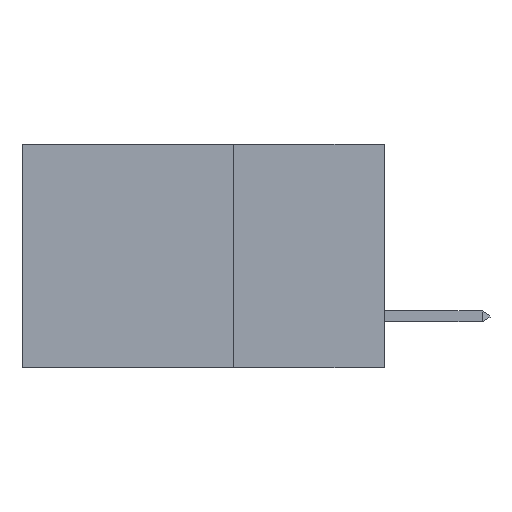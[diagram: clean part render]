
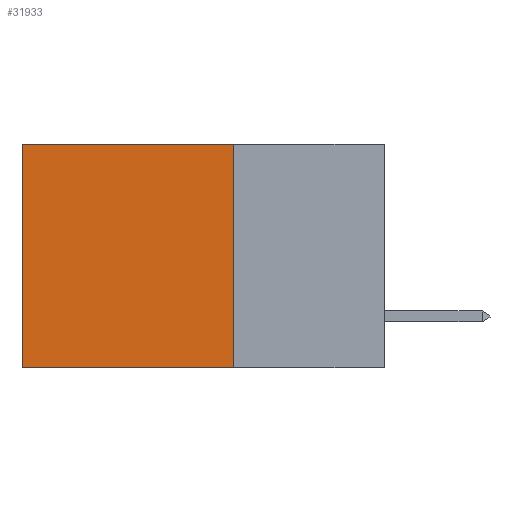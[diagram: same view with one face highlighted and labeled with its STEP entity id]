
A CAD part, left-side view. The second image highlights one B-rep face of the part: STEP entity #31933.
In plain terms, the highlighted planar face has unit normal (-1, 0, 0).
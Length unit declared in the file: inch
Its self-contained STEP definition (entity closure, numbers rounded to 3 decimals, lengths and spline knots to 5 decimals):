
#1397 = VERTEX_POINT ( 'NONE', #3713 ) ;
#1494 = DIRECTION ( 'NONE',  ( 0., 1., 0. ) ) ;
#3355 = DIRECTION ( 'NONE',  ( 0., 0., -1. ) ) ;
#3713 = CARTESIAN_POINT ( 'NONE',  ( 0.2875, 0.6, -0.37 ) ) ;
#4660 = VECTOR ( 'NONE', #1494, 39.37008 ) ;
#7984 = CARTESIAN_POINT ( 'NONE',  ( 0.2875, 0.6, 0. ) ) ;
#8040 = ORIENTED_EDGE ( 'NONE', *, *, #15448, .T. ) ;
#9040 = ORIENTED_EDGE ( 'NONE', *, *, #17969, .F. ) ;
#9834 = CARTESIAN_POINT ( 'NONE',  ( 0.2875, 0.25, -0.37 ) ) ;
#11094 = CARTESIAN_POINT ( 'NONE',  ( 0.2875, 0.6, 0. ) ) ;
#11198 = DIRECTION ( 'NONE',  ( 0., 0., -1. ) ) ;
#12249 = VERTEX_POINT ( 'NONE', #24648 ) ;
#13356 = VECTOR ( 'NONE', #24672, 39.37008 ) ;
#13552 = VECTOR ( 'NONE', #27266, 39.37008 ) ;
#14131 = CARTESIAN_POINT ( 'NONE',  ( 0.2875, 0.25, 0. ) ) ;
#14421 = LINE ( 'NONE', #35478, #13552 ) ;
#14727 = AXIS2_PLACEMENT_3D ( 'NONE', #25560, #20066, #3355 ) ;
#15448 = EDGE_CURVE ( 'NONE', #30072, #1397, #28113, .T. ) ;
#17969 = EDGE_CURVE ( 'NONE', #12249, #1397, #26944, .T. ) ;
#19619 = VERTEX_POINT ( 'NONE', #14131 ) ;
#20066 = DIRECTION ( 'NONE',  ( 1., 0., 0. ) ) ;
#22272 = CARTESIAN_POINT ( 'NONE',  ( 0.2875, 0.25, 0. ) ) ;
#24648 = CARTESIAN_POINT ( 'NONE',  ( 0.2875, 0.25, -0.37 ) ) ;
#24672 = DIRECTION ( 'NONE',  ( 0., 0., -1. ) ) ;
#25560 = CARTESIAN_POINT ( 'NONE',  ( 0.2875, 0.25, 0. ) ) ;
#25823 = EDGE_LOOP ( 'NONE', ( #8040, #9040, #28044, #31477 ) ) ;
#26645 = VECTOR ( 'NONE', #11198, 39.37008 ) ;
#26944 = LINE ( 'NONE', #9834, #4660 ) ;
#27266 = DIRECTION ( 'NONE',  ( 0., 1., 0. ) ) ;
#28044 = ORIENTED_EDGE ( 'NONE', *, *, #31815, .F. ) ;
#28113 = LINE ( 'NONE', #7984, #13356 ) ;
#30072 = VERTEX_POINT ( 'NONE', #11094 ) ;
#31111 = PLANE ( 'NONE',  #14727 ) ;
#31366 = FACE_OUTER_BOUND ( 'NONE', #25823, .T. ) ;
#31477 = ORIENTED_EDGE ( 'NONE', *, *, #32181, .T. ) ;
#31815 = EDGE_CURVE ( 'NONE', #19619, #12249, #33975, .T. ) ;
#31933 = ADVANCED_FACE ( 'NONE', ( #31366 ), #31111, .F. ) ;
#32181 = EDGE_CURVE ( 'NONE', #19619, #30072, #14421, .T. ) ;
#33975 = LINE ( 'NONE', #22272, #26645 ) ;
#35478 = CARTESIAN_POINT ( 'NONE',  ( 0.2875, 0.25, 0. ) ) ;
